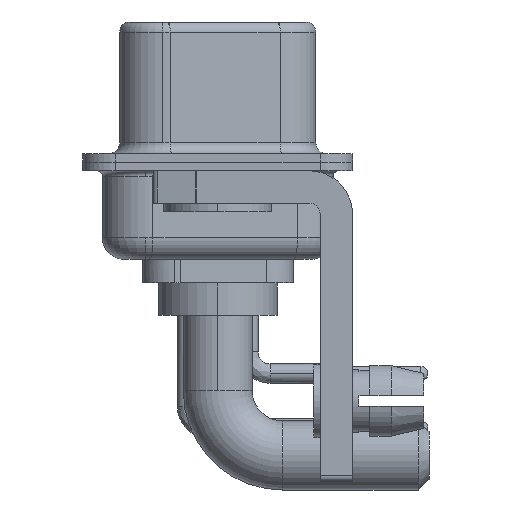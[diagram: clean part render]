
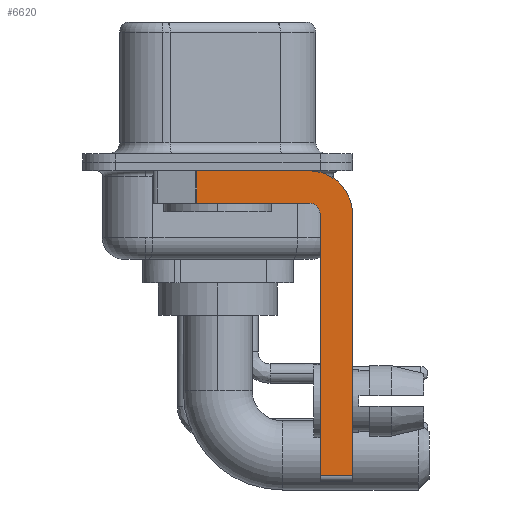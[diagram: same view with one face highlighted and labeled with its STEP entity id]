
A CAD part, left-side view. The second image highlights one B-rep face of the part: STEP entity #6620.
In plain terms, the highlighted planar face has unit normal (-1, 0, 0).
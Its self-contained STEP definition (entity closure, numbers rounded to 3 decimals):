
#205 = VERTEX_POINT ( 'NONE', #19321 ) ;
#430 = ORIENTED_EDGE ( 'NONE', *, *, #25566, .F. ) ;
#1424 = DIRECTION ( 'NONE',  ( 0., 0., -1. ) ) ;
#1926 = CIRCLE ( 'NONE', #17032, 0.5 ) ;
#2091 = VERTEX_POINT ( 'NONE', #21096 ) ;
#2151 = CIRCLE ( 'NONE', #7837, 2. ) ;
#2771 = DIRECTION ( 'NONE',  ( 0., 0., 1. ) ) ;
#3213 = CARTESIAN_POINT ( 'NONE',  ( -2.9, -4.25, -2.4 ) ) ;
#3967 = EDGE_CURVE ( 'NONE', #21496, #2091, #7401, .T. ) ;
#4002 = CARTESIAN_POINT ( 'NONE',  ( -2.9, -6.25, -2.4 ) ) ;
#4026 = ORIENTED_EDGE ( 'NONE', *, *, #28821, .F. ) ;
#5182 = CARTESIAN_POINT ( 'NONE',  ( -2.9, 3., -0.4 ) ) ;
#5669 = ORIENTED_EDGE ( 'NONE', *, *, #6076, .T. ) ;
#6076 = EDGE_CURVE ( 'NONE', #21496, #205, #14777, .T. ) ;
#6171 = EDGE_CURVE ( 'NONE', #2091, #9491, #2151, .T. ) ;
#6620 = ADVANCED_FACE ( 'NONE', ( #12686 ), #23894, .F. ) ;
#7401 = LINE ( 'NONE', #5182, #20910 ) ;
#7837 = AXIS2_PLACEMENT_3D ( 'NONE', #21994, #25977, #8288 ) ;
#8288 = DIRECTION ( 'NONE',  ( 0., 0., -1. ) ) ;
#8960 = LINE ( 'NONE', #13384, #19207 ) ;
#9487 = VERTEX_POINT ( 'NONE', #10658 ) ;
#9491 = VERTEX_POINT ( 'NONE', #4002 ) ;
#9697 = EDGE_CURVE ( 'NONE', #13652, #205, #8960, .T. ) ;
#9995 = LINE ( 'NONE', #14565, #16291 ) ;
#10654 = CARTESIAN_POINT ( 'NONE',  ( -2.9, -4.75, -2.4 ) ) ;
#10658 = CARTESIAN_POINT ( 'NONE',  ( -2.9, -6.25, -14.55 ) ) ;
#11622 = VECTOR ( 'NONE', #12582, 1000. ) ;
#11818 = EDGE_CURVE ( 'NONE', #26267, #9487, #24700, .T. ) ;
#11871 = EDGE_LOOP ( 'NONE', ( #24042, #5669, #20079, #20432, #4026, #23759, #430, #26148 ) ) ;
#12087 = DIRECTION ( 'NONE',  ( -1., 0., 0. ) ) ;
#12277 = CARTESIAN_POINT ( 'NONE',  ( -2.9, -4.25, -1.9 ) ) ;
#12582 = DIRECTION ( 'NONE',  ( 0., 0., -1. ) ) ;
#12686 = FACE_OUTER_BOUND ( 'NONE', #11871, .T. ) ;
#12977 = DIRECTION ( 'NONE',  ( 0., 0., -1. ) ) ;
#13384 = CARTESIAN_POINT ( 'NONE',  ( -2.9, -4.25, -1.9 ) ) ;
#13652 = VERTEX_POINT ( 'NONE', #12277 ) ;
#13799 = VERTEX_POINT ( 'NONE', #10654 ) ;
#14122 = DIRECTION ( 'NONE',  ( 0., 0., 1. ) ) ;
#14565 = CARTESIAN_POINT ( 'NONE',  ( -2.9, -4.75, -14.8 ) ) ;
#14777 = LINE ( 'NONE', #28632, #11622 ) ;
#14982 = VECTOR ( 'NONE', #24857, 1000. ) ;
#15157 = CARTESIAN_POINT ( 'NONE',  ( -2.9, -6.25, -2.4 ) ) ;
#15480 = EDGE_CURVE ( 'NONE', #13799, #13652, #1926, .T. ) ;
#16130 = AXIS2_PLACEMENT_3D ( 'NONE', #25948, #26379, #12977 ) ;
#16291 = VECTOR ( 'NONE', #14122, 1000. ) ;
#17032 = AXIS2_PLACEMENT_3D ( 'NONE', #3213, #12087, #2771 ) ;
#18349 = CARTESIAN_POINT ( 'NONE',  ( -2.9, -4.75, -14.55 ) ) ;
#19207 = VECTOR ( 'NONE', #19880, 1000. ) ;
#19321 = CARTESIAN_POINT ( 'NONE',  ( -2.9, 0.978, -1.9 ) ) ;
#19880 = DIRECTION ( 'NONE',  ( 0., 1., 0. ) ) ;
#20079 = ORIENTED_EDGE ( 'NONE', *, *, #9697, .F. ) ;
#20432 = ORIENTED_EDGE ( 'NONE', *, *, #15480, .F. ) ;
#20910 = VECTOR ( 'NONE', #21389, 1000. ) ;
#21096 = CARTESIAN_POINT ( 'NONE',  ( -2.9, -4.25, -0.4 ) ) ;
#21389 = DIRECTION ( 'NONE',  ( 0., -1., 0. ) ) ;
#21496 = VERTEX_POINT ( 'NONE', #27069 ) ;
#21646 = LINE ( 'NONE', #15157, #24214 ) ;
#21994 = CARTESIAN_POINT ( 'NONE',  ( -2.9, -4.25, -2.4 ) ) ;
#23759 = ORIENTED_EDGE ( 'NONE', *, *, #11818, .T. ) ;
#23894 = PLANE ( 'NONE',  #16130 ) ;
#24042 = ORIENTED_EDGE ( 'NONE', *, *, #3967, .F. ) ;
#24214 = VECTOR ( 'NONE', #1424, 1000. ) ;
#24700 = LINE ( 'NONE', #27049, #14982 ) ;
#24857 = DIRECTION ( 'NONE',  ( 0., -1., 0. ) ) ;
#25566 = EDGE_CURVE ( 'NONE', #9491, #9487, #21646, .T. ) ;
#25948 = CARTESIAN_POINT ( 'NONE',  ( -2.9, -4.25, -2.4 ) ) ;
#25977 = DIRECTION ( 'NONE',  ( 1., 0., 0. ) ) ;
#26148 = ORIENTED_EDGE ( 'NONE', *, *, #6171, .F. ) ;
#26267 = VERTEX_POINT ( 'NONE', #18349 ) ;
#26379 = DIRECTION ( 'NONE',  ( 1., 0., 0. ) ) ;
#27049 = CARTESIAN_POINT ( 'NONE',  ( -2.9, -4.25, -14.55 ) ) ;
#27069 = CARTESIAN_POINT ( 'NONE',  ( -2.9, 0.978, -0.4 ) ) ;
#28632 = CARTESIAN_POINT ( 'NONE',  ( -2.9, 0.978, -1.9 ) ) ;
#28821 = EDGE_CURVE ( 'NONE', #26267, #13799, #9995, .T. ) ;
